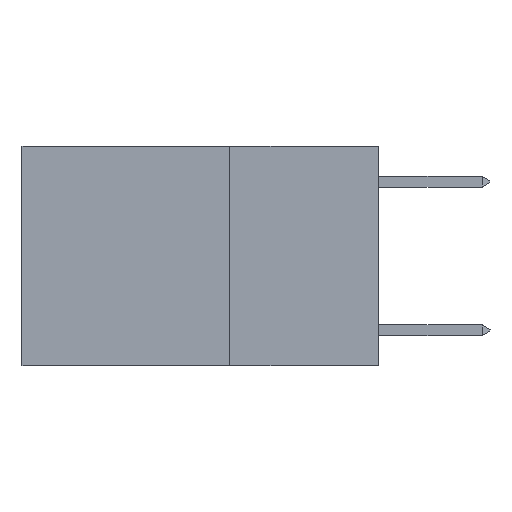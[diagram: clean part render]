
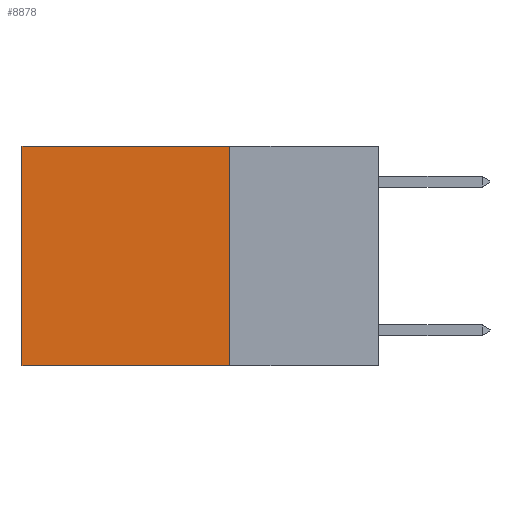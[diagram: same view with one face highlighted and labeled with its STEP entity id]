
A CAD part, left-side view. The second image highlights one B-rep face of the part: STEP entity #8878.
In plain terms, the highlighted planar face has unit normal (-1, 0, 0).
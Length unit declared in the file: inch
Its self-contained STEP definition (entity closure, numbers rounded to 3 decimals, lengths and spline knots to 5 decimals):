
#868 = CARTESIAN_POINT ( 'NONE',  ( 0.2625, 0.25, 0. ) ) ;
#1006 = LINE ( 'NONE', #25901, #1841 ) ;
#1841 = VECTOR ( 'NONE', #21325, 39.37008 ) ;
#2428 = FACE_OUTER_BOUND ( 'NONE', #29204, .T. ) ;
#3708 = LINE ( 'NONE', #16244, #27398 ) ;
#3988 = DIRECTION ( 'NONE',  ( 1., 0., 0. ) ) ;
#4162 = AXIS2_PLACEMENT_3D ( 'NONE', #18634, #3988, #11319 ) ;
#5140 = EDGE_CURVE ( 'NONE', #8226, #14220, #3708, .T. ) ;
#5950 = EDGE_CURVE ( 'NONE', #14220, #26046, #30864, .T. ) ;
#8226 = VERTEX_POINT ( 'NONE', #868 ) ;
#8399 = DIRECTION ( 'NONE',  ( 0., 0., -1. ) ) ;
#8878 = ADVANCED_FACE ( 'NONE', ( #2428 ), #12343, .F. ) ;
#9057 = DIRECTION ( 'NONE',  ( 0., 1., 0. ) ) ;
#10214 = DIRECTION ( 'NONE',  ( 0., 1., 0. ) ) ;
#10285 = VECTOR ( 'NONE', #10214, 39.37008 ) ;
#11319 = DIRECTION ( 'NONE',  ( 0., 0., -1. ) ) ;
#11342 = CARTESIAN_POINT ( 'NONE',  ( 0.2625, 0.6, 0. ) ) ;
#11779 = CARTESIAN_POINT ( 'NONE',  ( 0.2625, 0.6, -0.37 ) ) ;
#12343 = PLANE ( 'NONE',  #4162 ) ;
#12829 = CARTESIAN_POINT ( 'NONE',  ( 0.2625, 0.25, -0.37 ) ) ;
#13464 = ORIENTED_EDGE ( 'NONE', *, *, #21911, .F. ) ;
#14220 = VERTEX_POINT ( 'NONE', #21730 ) ;
#15103 = CARTESIAN_POINT ( 'NONE',  ( 0.2625, 0.25, -0.37 ) ) ;
#16244 = CARTESIAN_POINT ( 'NONE',  ( 0.2625, 0.25, 0. ) ) ;
#16901 = EDGE_CURVE ( 'NONE', #8226, #30516, #1006, .T. ) ;
#18009 = VECTOR ( 'NONE', #8399, 39.37008 ) ;
#18634 = CARTESIAN_POINT ( 'NONE',  ( 0.2625, 0.25, 0. ) ) ;
#21325 = DIRECTION ( 'NONE',  ( 0., 0., -1. ) ) ;
#21730 = CARTESIAN_POINT ( 'NONE',  ( 0.2625, 0.6, 0. ) ) ;
#21911 = EDGE_CURVE ( 'NONE', #30516, #26046, #25033, .T. ) ;
#23186 = ORIENTED_EDGE ( 'NONE', *, *, #5140, .T. ) ;
#25033 = LINE ( 'NONE', #12829, #10285 ) ;
#25901 = CARTESIAN_POINT ( 'NONE',  ( 0.2625, 0.25, 0. ) ) ;
#26046 = VERTEX_POINT ( 'NONE', #11779 ) ;
#27398 = VECTOR ( 'NONE', #9057, 39.37008 ) ;
#29204 = EDGE_LOOP ( 'NONE', ( #31827, #13464, #32080, #23186 ) ) ;
#30516 = VERTEX_POINT ( 'NONE', #15103 ) ;
#30864 = LINE ( 'NONE', #11342, #18009 ) ;
#31827 = ORIENTED_EDGE ( 'NONE', *, *, #5950, .T. ) ;
#32080 = ORIENTED_EDGE ( 'NONE', *, *, #16901, .F. ) ;
